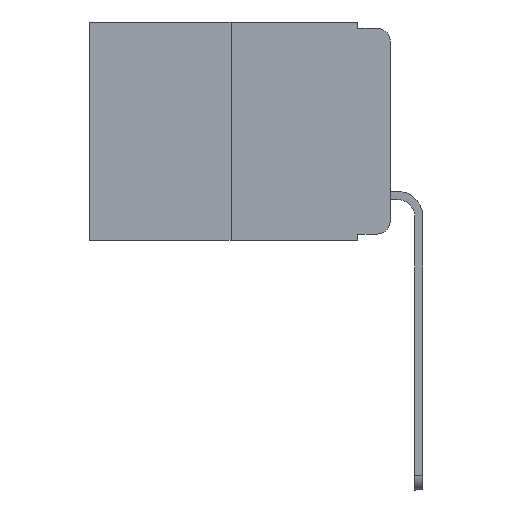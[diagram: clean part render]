
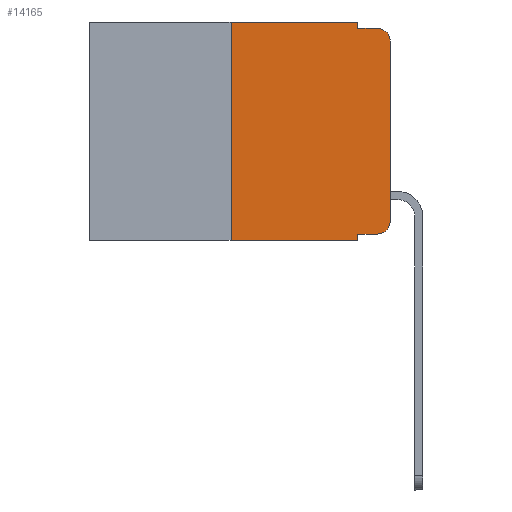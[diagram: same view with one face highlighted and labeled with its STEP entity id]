
A CAD part, left-side view. The second image highlights one B-rep face of the part: STEP entity #14165.
In plain terms, the highlighted planar face has unit normal (-1, 0, 0).
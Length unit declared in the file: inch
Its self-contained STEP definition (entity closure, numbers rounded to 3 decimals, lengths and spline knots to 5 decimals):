
#145 = CARTESIAN_POINT ( 'NONE',  ( 0., 0.25, 0. ) ) ;
#284 = CARTESIAN_POINT ( 'NONE',  ( 0., 0.051, -0.01 ) ) ;
#357 = LINE ( 'NONE', #14851, #2854 ) ;
#496 = DIRECTION ( 'NONE',  ( 0., -1., 0. ) ) ;
#509 = VECTOR ( 'NONE', #2564, 39.37008 ) ;
#696 = CARTESIAN_POINT ( 'NONE',  ( 0., 0., 0. ) ) ;
#1058 = VECTOR ( 'NONE', #11286, 39.37008 ) ;
#1387 = LINE ( 'NONE', #13355, #509 ) ;
#1423 = EDGE_CURVE ( 'NONE', #7594, #9611, #8767, .T. ) ;
#1604 = ORIENTED_EDGE ( 'NONE', *, *, #9271, .T. ) ;
#1678 = ORIENTED_EDGE ( 'NONE', *, *, #1423, .T. ) ;
#1824 = CARTESIAN_POINT ( 'NONE',  ( 0., 0.051, 0. ) ) ;
#1930 = DIRECTION ( 'NONE',  ( -1., 0., 0. ) ) ;
#2529 = DIRECTION ( 'NONE',  ( 0., 0., 1. ) ) ;
#2535 = ORIENTED_EDGE ( 'NONE', *, *, #13568, .F. ) ;
#2564 = DIRECTION ( 'NONE',  ( 0., 0., -1. ) ) ;
#2595 = CIRCLE ( 'NONE', #15157, 0.02 ) ;
#2687 = CARTESIAN_POINT ( 'NONE',  ( 0., 0.051, -0.333 ) ) ;
#2772 = VERTEX_POINT ( 'NONE', #12098 ) ;
#2854 = VECTOR ( 'NONE', #9832, 39.37008 ) ;
#2888 = ORIENTED_EDGE ( 'NONE', *, *, #4179, .T. ) ;
#3048 = VERTEX_POINT ( 'NONE', #11776 ) ;
#3859 = EDGE_CURVE ( 'NONE', #14111, #13697, #2595, .T. ) ;
#3949 = CARTESIAN_POINT ( 'NONE',  ( 0., 0.25, -0.343 ) ) ;
#4179 = EDGE_CURVE ( 'NONE', #7948, #2772, #14295, .T. ) ;
#4854 = CARTESIAN_POINT ( 'NONE',  ( 0., 0.02, -0.03 ) ) ;
#5325 = CARTESIAN_POINT ( 'NONE',  ( 0., 0.02, -0.313 ) ) ;
#5333 = EDGE_CURVE ( 'NONE', #14452, #13697, #357, .T. ) ;
#5593 = CARTESIAN_POINT ( 'NONE',  ( 0., 0., -0.03 ) ) ;
#5603 = CARTESIAN_POINT ( 'NONE',  ( 0., 0.051, 0. ) ) ;
#5754 = CARTESIAN_POINT ( 'NONE',  ( 0., 0.051, -0.343 ) ) ;
#5762 = AXIS2_PLACEMENT_3D ( 'NONE', #13292, #5979, #7179 ) ;
#5906 = ORIENTED_EDGE ( 'NONE', *, *, #14484, .T. ) ;
#5979 = DIRECTION ( 'NONE',  ( 1., 0., 0. ) ) ;
#6295 = VECTOR ( 'NONE', #12748, 39.37008 ) ;
#6422 = LINE ( 'NONE', #13805, #8748 ) ;
#6696 = VECTOR ( 'NONE', #2529, 39.37008 ) ;
#7179 = DIRECTION ( 'NONE',  ( 0., 0., -1. ) ) ;
#7537 = ORIENTED_EDGE ( 'NONE', *, *, #5333, .F. ) ;
#7594 = VERTEX_POINT ( 'NONE', #3949 ) ;
#7758 = AXIS2_PLACEMENT_3D ( 'NONE', #5325, #1930, #13905 ) ;
#7948 = VERTEX_POINT ( 'NONE', #15372 ) ;
#8001 = EDGE_CURVE ( 'NONE', #7594, #3048, #12068, .T. ) ;
#8122 = EDGE_LOOP ( 'NONE', ( #5906, #13147, #7537, #12517, #15089, #12274, #1678, #2535, #1604, #2888 ) ) ;
#8748 = VECTOR ( 'NONE', #496, 39.37008 ) ;
#8767 = LINE ( 'NONE', #8931, #1058 ) ;
#8931 = CARTESIAN_POINT ( 'NONE',  ( 0., 0.473, -0.343 ) ) ;
#9209 = LINE ( 'NONE', #696, #6295 ) ;
#9271 = EDGE_CURVE ( 'NONE', #10695, #7948, #12152, .T. ) ;
#9611 = VERTEX_POINT ( 'NONE', #5754 ) ;
#9832 = DIRECTION ( 'NONE',  ( 0., -1., 0. ) ) ;
#9976 = VECTOR ( 'NONE', #13402, 39.37008 ) ;
#10054 = VECTOR ( 'NONE', #14107, 39.37008 ) ;
#10348 = FACE_OUTER_BOUND ( 'NONE', #8122, .T. ) ;
#10695 = VERTEX_POINT ( 'NONE', #14419 ) ;
#10938 = DIRECTION ( 'NONE',  ( 0., 0., -1. ) ) ;
#11286 = DIRECTION ( 'NONE',  ( 0., -1., 0. ) ) ;
#11530 = LINE ( 'NONE', #5603, #10054 ) ;
#11732 = EDGE_CURVE ( 'NONE', #3048, #15247, #6422, .T. ) ;
#11776 = CARTESIAN_POINT ( 'NONE',  ( 0., 0.25, 0. ) ) ;
#11975 = CARTESIAN_POINT ( 'NONE',  ( 0., 0.02, -0.01 ) ) ;
#12041 = PLANE ( 'NONE',  #5762 ) ;
#12068 = LINE ( 'NONE', #145, #6696 ) ;
#12098 = CARTESIAN_POINT ( 'NONE',  ( 0., 0., -0.313 ) ) ;
#12152 = LINE ( 'NONE', #2687, #9976 ) ;
#12274 = ORIENTED_EDGE ( 'NONE', *, *, #8001, .F. ) ;
#12517 = ORIENTED_EDGE ( 'NONE', *, *, #14740, .F. ) ;
#12748 = DIRECTION ( 'NONE',  ( 0., 0., 1. ) ) ;
#13147 = ORIENTED_EDGE ( 'NONE', *, *, #3859, .T. ) ;
#13292 = CARTESIAN_POINT ( 'NONE',  ( 0., 0.473, 0. ) ) ;
#13355 = CARTESIAN_POINT ( 'NONE',  ( 0., 0.051, 0. ) ) ;
#13402 = DIRECTION ( 'NONE',  ( 0., -1., 0. ) ) ;
#13568 = EDGE_CURVE ( 'NONE', #10695, #9611, #11530, .T. ) ;
#13697 = VERTEX_POINT ( 'NONE', #11975 ) ;
#13805 = CARTESIAN_POINT ( 'NONE',  ( 0., 0.473, 0. ) ) ;
#13905 = DIRECTION ( 'NONE',  ( 0., 0., -1. ) ) ;
#14107 = DIRECTION ( 'NONE',  ( 0., 0., -1. ) ) ;
#14111 = VERTEX_POINT ( 'NONE', #5593 ) ;
#14158 = DIRECTION ( 'NONE',  ( -1., 0., 0. ) ) ;
#14165 = ADVANCED_FACE ( 'NONE', ( #10348 ), #12041, .F. ) ;
#14295 = CIRCLE ( 'NONE', #7758, 0.02 ) ;
#14419 = CARTESIAN_POINT ( 'NONE',  ( 0., 0.051, -0.333 ) ) ;
#14452 = VERTEX_POINT ( 'NONE', #284 ) ;
#14484 = EDGE_CURVE ( 'NONE', #2772, #14111, #9209, .T. ) ;
#14740 = EDGE_CURVE ( 'NONE', #15247, #14452, #1387, .T. ) ;
#14851 = CARTESIAN_POINT ( 'NONE',  ( 0., 0.051, -0.01 ) ) ;
#15089 = ORIENTED_EDGE ( 'NONE', *, *, #11732, .F. ) ;
#15157 = AXIS2_PLACEMENT_3D ( 'NONE', #4854, #14158, #10938 ) ;
#15247 = VERTEX_POINT ( 'NONE', #1824 ) ;
#15372 = CARTESIAN_POINT ( 'NONE',  ( 0., 0.02, -0.333 ) ) ;
